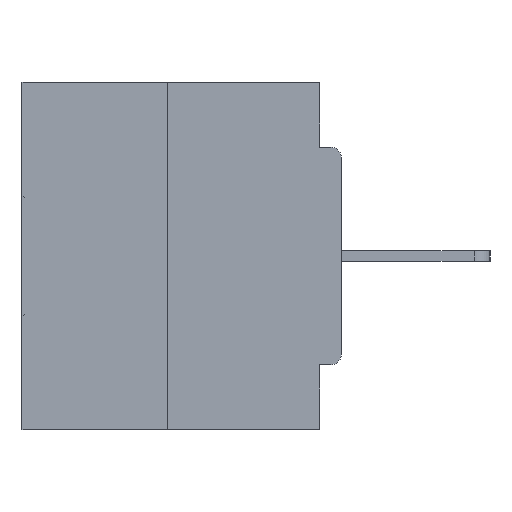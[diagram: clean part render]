
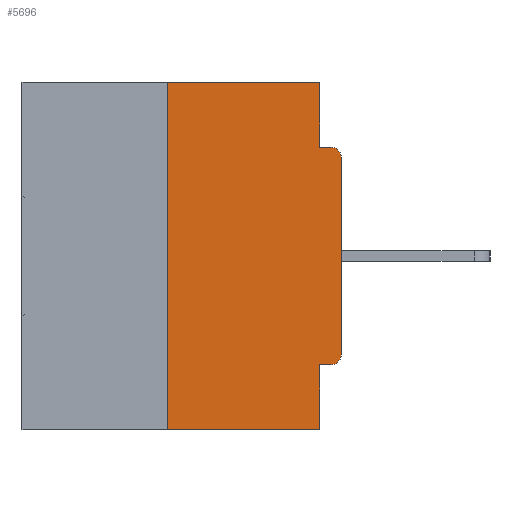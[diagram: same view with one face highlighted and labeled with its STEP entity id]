
A CAD part, left-side view. The second image highlights one B-rep face of the part: STEP entity #5696.
In plain terms, the highlighted planar face has unit normal (-1, 0, 0).
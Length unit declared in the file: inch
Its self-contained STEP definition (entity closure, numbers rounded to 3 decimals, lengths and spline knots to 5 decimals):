
#918 = ORIENTED_EDGE ( 'NONE', *, *, #2386, .T. ) ;
#1782 = EDGE_CURVE ( 'NONE', #23064, #20700, #20726, .T. ) ;
#2261 = DIRECTION ( 'NONE',  ( 0., 1., 0. ) ) ;
#2386 = EDGE_CURVE ( 'NONE', #14547, #14720, #25584, .T. ) ;
#2544 = VECTOR ( 'NONE', #22663, 39.37008 ) ;
#4202 = DIRECTION ( 'NONE',  ( 0., 0., 1. ) ) ;
#4261 = ORIENTED_EDGE ( 'NONE', *, *, #20838, .F. ) ;
#5530 = ORIENTED_EDGE ( 'NONE', *, *, #20472, .F. ) ;
#5696 = ADVANCED_FACE ( 'NONE', ( #28794 ), #26114, .F. ) ;
#6419 = CARTESIAN_POINT ( 'NONE',  ( 0., 0., -0.0935 ) ) ;
#7054 = VERTEX_POINT ( 'NONE', #27220 ) ;
#7189 = DIRECTION ( 'NONE',  ( 0., -1., 0. ) ) ;
#8206 = EDGE_CURVE ( 'NONE', #29417, #14893, #31274, .T. ) ;
#8403 = EDGE_LOOP ( 'NONE', ( #22784, #4261, #24326, #13936, #5530, #918, #8450, #11556, #33984, #10147 ) ) ;
#8450 = ORIENTED_EDGE ( 'NONE', *, *, #9077, .T. ) ;
#8517 = DIRECTION ( 'NONE',  ( -1., 0., 0. ) ) ;
#9077 = EDGE_CURVE ( 'NONE', #14720, #14890, #28362, .T. ) ;
#9404 = CARTESIAN_POINT ( 'NONE',  ( 0., 0., -0.3915 ) ) ;
#9660 = LINE ( 'NONE', #29052, #22085 ) ;
#9704 = CARTESIAN_POINT ( 'NONE',  ( 0., 0., -0.4065 ) ) ;
#9873 = CARTESIAN_POINT ( 'NONE',  ( 0., 0.46, -0.5 ) ) ;
#10147 = ORIENTED_EDGE ( 'NONE', *, *, #8206, .F. ) ;
#10444 = VECTOR ( 'NONE', #16536, 39.37008 ) ;
#11006 = CARTESIAN_POINT ( 'NONE',  ( 0., 0.015, -0.4065 ) ) ;
#11368 = LINE ( 'NONE', #6419, #10444 ) ;
#11556 = ORIENTED_EDGE ( 'NONE', *, *, #23850, .T. ) ;
#12025 = LINE ( 'NONE', #9704, #31994 ) ;
#12154 = CARTESIAN_POINT ( 'NONE',  ( 0., 0.015, -0.1085 ) ) ;
#12243 = DIRECTION ( 'NONE',  ( 0., 0., -1. ) ) ;
#12577 = CARTESIAN_POINT ( 'NONE',  ( 0., 0., -0.1085 ) ) ;
#12582 = DIRECTION ( 'NONE',  ( 1., 0., 0. ) ) ;
#12628 = LINE ( 'NONE', #23491, #2544 ) ;
#13577 = VECTOR ( 'NONE', #15911, 39.37008 ) ;
#13936 = ORIENTED_EDGE ( 'NONE', *, *, #24230, .F. ) ;
#14547 = VERTEX_POINT ( 'NONE', #11006 ) ;
#14720 = VERTEX_POINT ( 'NONE', #9404 ) ;
#14890 = VERTEX_POINT ( 'NONE', #12577 ) ;
#14893 = VERTEX_POINT ( 'NONE', #21481 ) ;
#15102 = CARTESIAN_POINT ( 'NONE',  ( 0., 0.031, -0.5 ) ) ;
#15103 = CARTESIAN_POINT ( 'NONE',  ( 0., 0.031, 0. ) ) ;
#15348 = AXIS2_PLACEMENT_3D ( 'NONE', #22042, #8517, #33241 ) ;
#15911 = DIRECTION ( 'NONE',  ( 0., -1., 0. ) ) ;
#16128 = VECTOR ( 'NONE', #12243, 39.37008 ) ;
#16536 = DIRECTION ( 'NONE',  ( 0., -1., 0. ) ) ;
#17835 = CARTESIAN_POINT ( 'NONE',  ( 0., 0., 0. ) ) ;
#18202 = CARTESIAN_POINT ( 'NONE',  ( 0., 0.031, 0. ) ) ;
#18624 = VERTEX_POINT ( 'NONE', #21062 ) ;
#18965 = CARTESIAN_POINT ( 'NONE',  ( 0., 0.25, -0.5 ) ) ;
#20096 = CIRCLE ( 'NONE', #25764, 0.015 ) ;
#20472 = EDGE_CURVE ( 'NONE', #14547, #18624, #12025, .T. ) ;
#20700 = VERTEX_POINT ( 'NONE', #24621 ) ;
#20726 = LINE ( 'NONE', #9873, #13577 ) ;
#20838 = EDGE_CURVE ( 'NONE', #23064, #24776, #12628, .T. ) ;
#20999 = EDGE_CURVE ( 'NONE', #14893, #7054, #11368, .T. ) ;
#21062 = CARTESIAN_POINT ( 'NONE',  ( 0., 0.031, -0.4065 ) ) ;
#21481 = CARTESIAN_POINT ( 'NONE',  ( 0., 0.031, -0.0935 ) ) ;
#22042 = CARTESIAN_POINT ( 'NONE',  ( 0., 0.015, -0.3915 ) ) ;
#22085 = VECTOR ( 'NONE', #7189, 39.37008 ) ;
#22663 = DIRECTION ( 'NONE',  ( 0., 0., 1. ) ) ;
#22784 = ORIENTED_EDGE ( 'NONE', *, *, #25246, .F. ) ;
#23064 = VERTEX_POINT ( 'NONE', #18965 ) ;
#23388 = CARTESIAN_POINT ( 'NONE',  ( 0., 0.25, 0. ) ) ;
#23491 = CARTESIAN_POINT ( 'NONE',  ( 0., 0.25, 0. ) ) ;
#23850 = EDGE_CURVE ( 'NONE', #14890, #7054, #20096, .T. ) ;
#24230 = EDGE_CURVE ( 'NONE', #18624, #20700, #27608, .T. ) ;
#24326 = ORIENTED_EDGE ( 'NONE', *, *, #1782, .T. ) ;
#24459 = AXIS2_PLACEMENT_3D ( 'NONE', #26825, #12582, #31614 ) ;
#24621 = CARTESIAN_POINT ( 'NONE',  ( 0., 0.031, -0.5 ) ) ;
#24776 = VERTEX_POINT ( 'NONE', #23388 ) ;
#25246 = EDGE_CURVE ( 'NONE', #24776, #29417, #9660, .T. ) ;
#25584 = CIRCLE ( 'NONE', #15348, 0.015 ) ;
#25764 = AXIS2_PLACEMENT_3D ( 'NONE', #12154, #31696, #28699 ) ;
#25944 = DIRECTION ( 'NONE',  ( 0., 0., -1. ) ) ;
#26114 = PLANE ( 'NONE',  #24459 ) ;
#26825 = CARTESIAN_POINT ( 'NONE',  ( 0., 0.46, 0. ) ) ;
#26857 = VECTOR ( 'NONE', #25944, 39.37008 ) ;
#26973 = VECTOR ( 'NONE', #4202, 39.37008 ) ;
#27220 = CARTESIAN_POINT ( 'NONE',  ( 0., 0.015, -0.0935 ) ) ;
#27608 = LINE ( 'NONE', #15102, #16128 ) ;
#28362 = LINE ( 'NONE', #17835, #26973 ) ;
#28699 = DIRECTION ( 'NONE',  ( 0., 0., -1. ) ) ;
#28794 = FACE_OUTER_BOUND ( 'NONE', #8403, .T. ) ;
#29052 = CARTESIAN_POINT ( 'NONE',  ( 0., 0.46, 0. ) ) ;
#29417 = VERTEX_POINT ( 'NONE', #18202 ) ;
#31274 = LINE ( 'NONE', #15103, #26857 ) ;
#31614 = DIRECTION ( 'NONE',  ( 0., 0., -1. ) ) ;
#31696 = DIRECTION ( 'NONE',  ( -1., 0., 0. ) ) ;
#31994 = VECTOR ( 'NONE', #2261, 39.37008 ) ;
#33241 = DIRECTION ( 'NONE',  ( 0., 0., -1. ) ) ;
#33984 = ORIENTED_EDGE ( 'NONE', *, *, #20999, .F. ) ;
